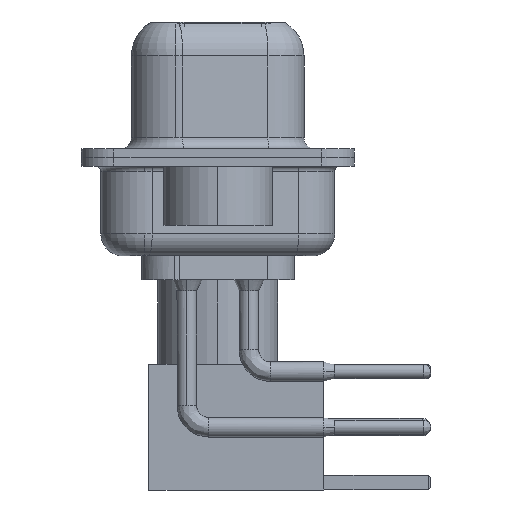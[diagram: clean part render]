
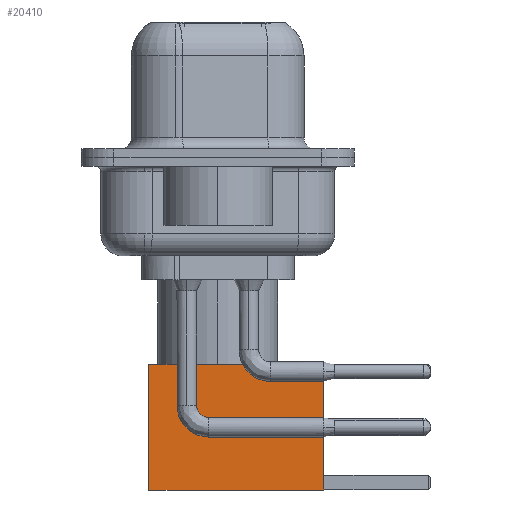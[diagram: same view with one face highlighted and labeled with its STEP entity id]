
A CAD part, left-side view. The second image highlights one B-rep face of the part: STEP entity #20410.
In plain terms, the highlighted face is planar.
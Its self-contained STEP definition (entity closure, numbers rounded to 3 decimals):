
#3063 = DIRECTION ( 'NONE',  ( 0., 1., 0. ) ) ;
#3612 = CARTESIAN_POINT ( 'NONE',  ( 2.875, 2.875, 8. ) ) ;
#4489 = EDGE_CURVE ( 'NONE', #6983, #12075, #9557, .T. ) ;
#4633 = CARTESIAN_POINT ( 'NONE',  ( 0., 2.875, 0. ) ) ;
#6983 = VERTEX_POINT ( 'NONE', #3612 ) ;
#7227 = EDGE_CURVE ( 'NONE', #17455, #15434, #25390, .T. ) ;
#8466 = VECTOR ( 'NONE', #23119, 1000. ) ;
#8483 = CARTESIAN_POINT ( 'NONE',  ( 2.875, 2.875, 0. ) ) ;
#8495 = VECTOR ( 'NONE', #13158, 1000. ) ;
#8754 = VECTOR ( 'NONE', #10363, 1000. ) ;
#9424 = VECTOR ( 'NONE', #19562, 1000. ) ;
#9557 = LINE ( 'NONE', #19696, #9424 ) ;
#10230 = CARTESIAN_POINT ( 'NONE',  ( -2.875, 2.875, 0. ) ) ;
#10363 = DIRECTION ( 'NONE',  ( -1., 0., 0. ) ) ;
#11428 = EDGE_CURVE ( 'NONE', #12075, #15434, #24419, .T. ) ;
#12075 = VERTEX_POINT ( 'NONE', #8483 ) ;
#13158 = DIRECTION ( 'NONE',  ( 0., 0., -1. ) ) ;
#13212 = DIRECTION ( 'NONE',  ( 0., 0., 1. ) ) ;
#13617 = ORIENTED_EDGE ( 'NONE', *, *, #17061, .F. ) ;
#13954 = ORIENTED_EDGE ( 'NONE', *, *, #7227, .F. ) ;
#14689 = ORIENTED_EDGE ( 'NONE', *, *, #11428, .T. ) ;
#14792 = FACE_OUTER_BOUND ( 'NONE', #24981, .T. ) ;
#15434 = VERTEX_POINT ( 'NONE', #10230 ) ;
#15624 = CARTESIAN_POINT ( 'NONE',  ( -2.875, 2.875, 0. ) ) ;
#17061 = EDGE_CURVE ( 'NONE', #6983, #17455, #21149, .T. ) ;
#17455 = VERTEX_POINT ( 'NONE', #22193 ) ;
#18821 = PLANE ( 'NONE',  #24950 ) ;
#19562 = DIRECTION ( 'NONE',  ( 0., 0., -1. ) ) ;
#19696 = CARTESIAN_POINT ( 'NONE',  ( 2.875, 2.875, 0. ) ) ;
#20410 = ADVANCED_FACE ( 'NONE', ( #14792 ), #18821, .T. ) ;
#21149 = LINE ( 'NONE', #23379, #8466 ) ;
#22193 = CARTESIAN_POINT ( 'NONE',  ( -2.875, 2.875, 8. ) ) ;
#22680 = ORIENTED_EDGE ( 'NONE', *, *, #4489, .T. ) ;
#22993 = CARTESIAN_POINT ( 'NONE',  ( 2.875, 2.875, 0. ) ) ;
#23119 = DIRECTION ( 'NONE',  ( -1., 0., 0. ) ) ;
#23379 = CARTESIAN_POINT ( 'NONE',  ( 0., 2.875, 8. ) ) ;
#24419 = LINE ( 'NONE', #4633, #8754 ) ;
#24950 = AXIS2_PLACEMENT_3D ( 'NONE', #22993, #3063, #13212 ) ;
#24981 = EDGE_LOOP ( 'NONE', ( #22680, #14689, #13954, #13617 ) ) ;
#25390 = LINE ( 'NONE', #15624, #8495 ) ;
